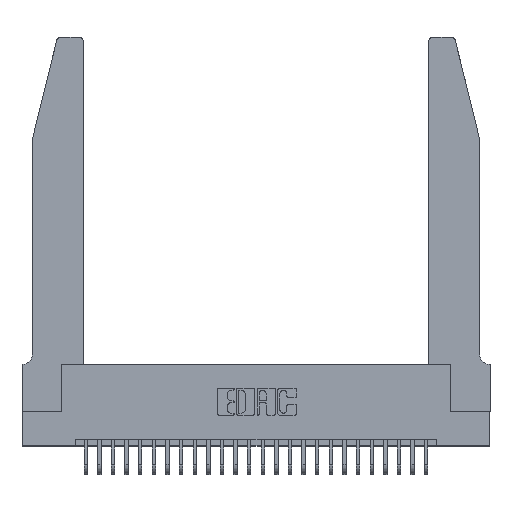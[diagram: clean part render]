
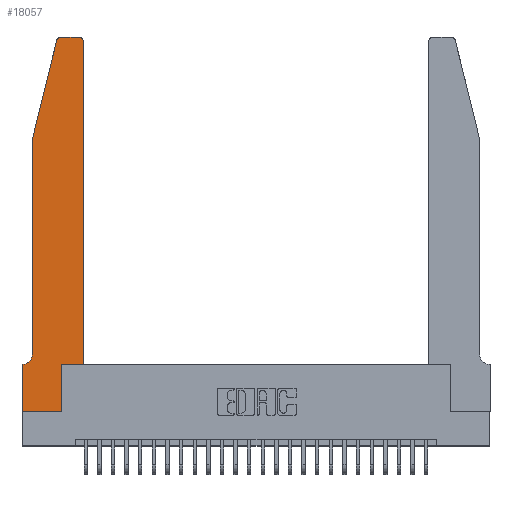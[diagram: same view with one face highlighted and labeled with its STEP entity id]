
A CAD part, top view. The second image highlights one B-rep face of the part: STEP entity #18057.
In plain terms, the highlighted planar face has unit normal (0, 0, 1).
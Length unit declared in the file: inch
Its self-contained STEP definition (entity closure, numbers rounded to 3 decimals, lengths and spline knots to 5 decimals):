
#78 = CARTESIAN_POINT ( 'NONE',  ( 0.284, 2.72, 0.37 ) ) ;
#84 = EDGE_CURVE ( 'NONE', #24011, #17994, #25594, .T. ) ;
#614 = CARTESIAN_POINT ( 'NONE',  ( 0.4205, 2.75, 0.37 ) ) ;
#660 = VECTOR ( 'NONE', #11472, 39.37008 ) ;
#1014 = LINE ( 'NONE', #9187, #660 ) ;
#1251 = LINE ( 'NONE', #27333, #5803 ) ;
#1269 = ORIENTED_EDGE ( 'NONE', *, *, #12831, .T. ) ;
#1488 = DIRECTION ( 'NONE',  ( 0., 1., 0. ) ) ;
#1712 = ORIENTED_EDGE ( 'NONE', *, *, #27985, .T. ) ;
#2189 = LINE ( 'NONE', #22206, #23240 ) ;
#2521 = ORIENTED_EDGE ( 'NONE', *, *, #22748, .T. ) ;
#2593 = CARTESIAN_POINT ( 'NONE',  ( 0.0055, 0.35, 0.37 ) ) ;
#2763 = EDGE_CURVE ( 'NONE', #19996, #15148, #19622, .T. ) ;
#2937 = EDGE_CURVE ( 'NONE', #23489, #19996, #1014, .T. ) ;
#3452 = CARTESIAN_POINT ( 'NONE',  ( 0.0755, 2., 0.37 ) ) ;
#4180 = VECTOR ( 'NONE', #1488, 39.37008 ) ;
#4271 = DIRECTION ( 'NONE',  ( 0., -1., 0. ) ) ;
#4312 = EDGE_LOOP ( 'NONE', ( #2521, #11774, #1269, #25000, #24516, #23866, #24527, #23717, #25538, #1712, #5521, #7881 ) ) ;
#4369 = PLANE ( 'NONE',  #12815 ) ;
#4580 = VECTOR ( 'NONE', #25032, 39.37008 ) ;
#5119 = EDGE_CURVE ( 'NONE', #9320, #28783, #17372, .T. ) ;
#5521 = ORIENTED_EDGE ( 'NONE', *, *, #22449, .T. ) ;
#5803 = VECTOR ( 'NONE', #7655, 39.37008 ) ;
#6216 = CARTESIAN_POINT ( 'NONE',  ( 0.0755, 0.42, 0.37 ) ) ;
#6323 = AXIS2_PLACEMENT_3D ( 'NONE', #78, #28837, #20279 ) ;
#7328 = DIRECTION ( 'NONE',  ( 1., 0., 0. ) ) ;
#7430 = DIRECTION ( 'NONE',  ( 0., 0., -1. ) ) ;
#7655 = DIRECTION ( 'NONE',  ( 1., 0., 0. ) ) ;
#7881 = ORIENTED_EDGE ( 'NONE', *, *, #12129, .T. ) ;
#8292 = CARTESIAN_POINT ( 'NONE',  ( 0.0755, 0.35, 0.37 ) ) ;
#8566 = VECTOR ( 'NONE', #11913, 39.37008 ) ;
#9187 = CARTESIAN_POINT ( 'NONE',  ( 0., 0., 0.37 ) ) ;
#9320 = VERTEX_POINT ( 'NONE', #17656 ) ;
#9473 = DIRECTION ( 'NONE',  ( 0., 0., 1. ) ) ;
#10746 = CARTESIAN_POINT ( 'NONE',  ( 0.4505, 2.72, 0.37 ) ) ;
#10906 = LINE ( 'NONE', #8292, #4580 ) ;
#11043 = LINE ( 'NONE', #22598, #25073 ) ;
#11116 = VERTEX_POINT ( 'NONE', #10746 ) ;
#11236 = CARTESIAN_POINT ( 'NONE',  ( 0., 0.35, 0.37 ) ) ;
#11472 = DIRECTION ( 'NONE',  ( 1., 0., 0. ) ) ;
#11727 = VERTEX_POINT ( 'NONE', #28326 ) ;
#11774 = ORIENTED_EDGE ( 'NONE', *, *, #5119, .T. ) ;
#11913 = DIRECTION ( 'NONE',  ( -1., 0., 0. ) ) ;
#12129 = EDGE_CURVE ( 'NONE', #11116, #27990, #19464, .T. ) ;
#12815 = AXIS2_PLACEMENT_3D ( 'NONE', #11236, #20062, #20159 ) ;
#12831 = EDGE_CURVE ( 'NONE', #28783, #24566, #22217, .T. ) ;
#13299 = CARTESIAN_POINT ( 'NONE',  ( 0., 0., 0.37 ) ) ;
#13452 = EDGE_CURVE ( 'NONE', #24566, #24011, #2189, .T. ) ;
#13475 = DIRECTION ( 'NONE',  ( -0.239, -0.971, 0. ) ) ;
#15148 = VERTEX_POINT ( 'NONE', #24588 ) ;
#15822 = AXIS2_PLACEMENT_3D ( 'NONE', #20872, #7430, #23132 ) ;
#17372 = CIRCLE ( 'NONE', #6323, 0.03 ) ;
#17656 = CARTESIAN_POINT ( 'NONE',  ( 0.284, 2.75, 0.37 ) ) ;
#17986 = EDGE_CURVE ( 'NONE', #17994, #24956, #10906, .T. ) ;
#17994 = VERTEX_POINT ( 'NONE', #2593 ) ;
#18037 = VECTOR ( 'NONE', #13475, 39.37008 ) ;
#18057 = ADVANCED_FACE ( 'NONE', ( #28042 ), #4369, .T. ) ;
#18107 = LINE ( 'NONE', #28014, #28181 ) ;
#19349 = DIRECTION ( 'NONE',  ( 0., 1., 0. ) ) ;
#19464 = CIRCLE ( 'NONE', #24101, 0.03 ) ;
#19622 = LINE ( 'NONE', #26059, #4180 ) ;
#19996 = VERTEX_POINT ( 'NONE', #21589 ) ;
#20062 = DIRECTION ( 'NONE',  ( 0., 0., 1. ) ) ;
#20159 = DIRECTION ( 'NONE',  ( 1., 0., 0. ) ) ;
#20181 = CARTESIAN_POINT ( 'NONE',  ( 0.2605, 2.75, 0.37 ) ) ;
#20279 = DIRECTION ( 'NONE',  ( 1., 0., 0. ) ) ;
#20665 = CARTESIAN_POINT ( 'NONE',  ( 0.4205, 2.72, 0.37 ) ) ;
#20830 = CARTESIAN_POINT ( 'NONE',  ( 0.0755, 2., 0.37 ) ) ;
#20872 = CARTESIAN_POINT ( 'NONE',  ( 0.0055, 0.42, 0.37 ) ) ;
#21589 = CARTESIAN_POINT ( 'NONE',  ( 0.2865, 0., 0.37 ) ) ;
#21919 = CARTESIAN_POINT ( 'NONE',  ( 0.25487, 2.72718, 0.37 ) ) ;
#22206 = CARTESIAN_POINT ( 'NONE',  ( 0.0755, 2., 0.37 ) ) ;
#22217 = LINE ( 'NONE', #20830, #18037 ) ;
#22229 = EDGE_CURVE ( 'NONE', #24956, #23489, #11043, .T. ) ;
#22449 = EDGE_CURVE ( 'NONE', #11727, #11116, #18107, .T. ) ;
#22598 = CARTESIAN_POINT ( 'NONE',  ( 0., 0., 0.37 ) ) ;
#22748 = EDGE_CURVE ( 'NONE', #27990, #9320, #23660, .T. ) ;
#22795 = DIRECTION ( 'NONE',  ( 0., -1., 0. ) ) ;
#23132 = DIRECTION ( 'NONE',  ( -1., 0., 0. ) ) ;
#23139 = CARTESIAN_POINT ( 'NONE',  ( 0., 0.35, 0.37 ) ) ;
#23240 = VECTOR ( 'NONE', #4271, 39.37008 ) ;
#23489 = VERTEX_POINT ( 'NONE', #13299 ) ;
#23660 = LINE ( 'NONE', #20181, #8566 ) ;
#23717 = ORIENTED_EDGE ( 'NONE', *, *, #2937, .T. ) ;
#23866 = ORIENTED_EDGE ( 'NONE', *, *, #17986, .T. ) ;
#24011 = VERTEX_POINT ( 'NONE', #6216 ) ;
#24101 = AXIS2_PLACEMENT_3D ( 'NONE', #20665, #9473, #7328 ) ;
#24516 = ORIENTED_EDGE ( 'NONE', *, *, #84, .T. ) ;
#24527 = ORIENTED_EDGE ( 'NONE', *, *, #22229, .T. ) ;
#24566 = VERTEX_POINT ( 'NONE', #3452 ) ;
#24588 = CARTESIAN_POINT ( 'NONE',  ( 0.2865, 0.35, 0.37 ) ) ;
#24956 = VERTEX_POINT ( 'NONE', #23139 ) ;
#25000 = ORIENTED_EDGE ( 'NONE', *, *, #13452, .T. ) ;
#25032 = DIRECTION ( 'NONE',  ( -1., 0., 0. ) ) ;
#25073 = VECTOR ( 'NONE', #22795, 39.37008 ) ;
#25538 = ORIENTED_EDGE ( 'NONE', *, *, #2763, .T. ) ;
#25594 = CIRCLE ( 'NONE', #15822, 0.07 ) ;
#26059 = CARTESIAN_POINT ( 'NONE',  ( 0.2865, 0.35, 0.37 ) ) ;
#27333 = CARTESIAN_POINT ( 'NONE',  ( 0.4505, 0.35, 0.37 ) ) ;
#27985 = EDGE_CURVE ( 'NONE', #15148, #11727, #1251, .T. ) ;
#27990 = VERTEX_POINT ( 'NONE', #614 ) ;
#28014 = CARTESIAN_POINT ( 'NONE',  ( 0.4505, 0.35, 0.37 ) ) ;
#28042 = FACE_OUTER_BOUND ( 'NONE', #4312, .T. ) ;
#28181 = VECTOR ( 'NONE', #19349, 39.37008 ) ;
#28326 = CARTESIAN_POINT ( 'NONE',  ( 0.4505, 0.35, 0.37 ) ) ;
#28783 = VERTEX_POINT ( 'NONE', #21919 ) ;
#28837 = DIRECTION ( 'NONE',  ( 0., 0., 1. ) ) ;
